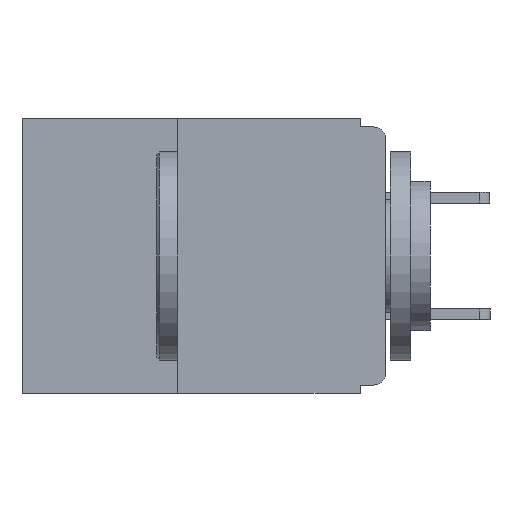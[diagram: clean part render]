
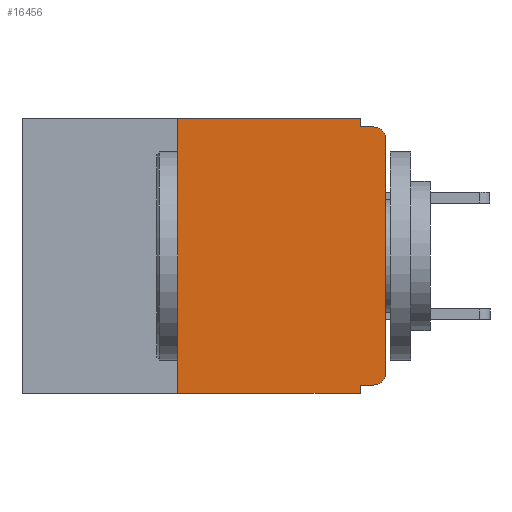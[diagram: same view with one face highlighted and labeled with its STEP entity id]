
A CAD part, left-side view. The second image highlights one B-rep face of the part: STEP entity #16456.
In plain terms, the highlighted planar face has unit normal (-1, 0, 0).
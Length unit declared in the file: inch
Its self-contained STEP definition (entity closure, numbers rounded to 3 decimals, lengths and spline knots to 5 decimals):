
#12 = EDGE_CURVE ( 'NONE', #5879, #13199, #8867, .T. ) ;
#127 = DIRECTION ( 'NONE',  ( -1., 0., 0. ) ) ;
#470 = CARTESIAN_POINT ( 'NONE',  ( 0., 0.031, -0.01 ) ) ;
#661 = CIRCLE ( 'NONE', #15094, 0.015 ) ;
#1228 = CARTESIAN_POINT ( 'NONE',  ( 0., 0.437, -0.33 ) ) ;
#1317 = DIRECTION ( 'NONE',  ( 1., 0., 0. ) ) ;
#1922 = VECTOR ( 'NONE', #11821, 39.37008 ) ;
#2860 = ORIENTED_EDGE ( 'NONE', *, *, #17256, .F. ) ;
#2930 = CARTESIAN_POINT ( 'NONE',  ( 0., 0., 0. ) ) ;
#3651 = VECTOR ( 'NONE', #21465, 39.37008 ) ;
#4110 = DIRECTION ( 'NONE',  ( 0., 0., -1. ) ) ;
#4394 = CARTESIAN_POINT ( 'NONE',  ( 0., 0.015, -0.025 ) ) ;
#4714 = CARTESIAN_POINT ( 'NONE',  ( 0., 0.015, -0.01 ) ) ;
#5103 = CARTESIAN_POINT ( 'NONE',  ( 0., 0.031, -0.33 ) ) ;
#5596 = CARTESIAN_POINT ( 'NONE',  ( 0., 0.25, -0.33 ) ) ;
#5879 = VERTEX_POINT ( 'NONE', #21097 ) ;
#6270 = VERTEX_POINT ( 'NONE', #7501 ) ;
#6344 = DIRECTION ( 'NONE',  ( 0., 0., -1. ) ) ;
#6626 = VECTOR ( 'NONE', #9047, 39.37008 ) ;
#7061 = CARTESIAN_POINT ( 'NONE',  ( 0., 0., -0.01 ) ) ;
#7126 = FACE_OUTER_BOUND ( 'NONE', #15646, .T. ) ;
#7146 = DIRECTION ( 'NONE',  ( 0., -1., 0. ) ) ;
#7501 = CARTESIAN_POINT ( 'NONE',  ( 0., 0., -0.305 ) ) ;
#7836 = EDGE_CURVE ( 'NONE', #10097, #23641, #9971, .T. ) ;
#7863 = CIRCLE ( 'NONE', #21084, 0.015 ) ;
#8867 = LINE ( 'NONE', #21626, #3651 ) ;
#8959 = LINE ( 'NONE', #16538, #19299 ) ;
#9010 = ORIENTED_EDGE ( 'NONE', *, *, #12, .F. ) ;
#9047 = DIRECTION ( 'NONE',  ( 0., -1., 0. ) ) ;
#9435 = EDGE_CURVE ( 'NONE', #13199, #20300, #24879, .T. ) ;
#9504 = DIRECTION ( 'NONE',  ( 0., 0., 1. ) ) ;
#9971 = LINE ( 'NONE', #7061, #24663 ) ;
#9978 = EDGE_CURVE ( 'NONE', #22343, #18645, #12930, .T. ) ;
#10097 = VERTEX_POINT ( 'NONE', #470 ) ;
#10645 = CARTESIAN_POINT ( 'NONE',  ( 0., 0., -0.025 ) ) ;
#10680 = DIRECTION ( 'NONE',  ( 0., 0., -1. ) ) ;
#11025 = PLANE ( 'NONE',  #11120 ) ;
#11120 = AXIS2_PLACEMENT_3D ( 'NONE', #24417, #1317, #14962 ) ;
#11288 = CARTESIAN_POINT ( 'NONE',  ( 0., 0.031, -0.32 ) ) ;
#11643 = VERTEX_POINT ( 'NONE', #20158 ) ;
#11813 = CARTESIAN_POINT ( 'NONE',  ( 0., 0.015, -0.305 ) ) ;
#11821 = DIRECTION ( 'NONE',  ( 0., -1., 0. ) ) ;
#11960 = ORIENTED_EDGE ( 'NONE', *, *, #9978, .F. ) ;
#12430 = LINE ( 'NONE', #2930, #13016 ) ;
#12455 = ORIENTED_EDGE ( 'NONE', *, *, #21321, .T. ) ;
#12930 = LINE ( 'NONE', #23226, #1922 ) ;
#13016 = VECTOR ( 'NONE', #16585, 39.37008 ) ;
#13199 = VERTEX_POINT ( 'NONE', #11288 ) ;
#13505 = ORIENTED_EDGE ( 'NONE', *, *, #15676, .T. ) ;
#13776 = DIRECTION ( 'NONE',  ( 0., 0., -1. ) ) ;
#14694 = EDGE_CURVE ( 'NONE', #11643, #20300, #22144, .T. ) ;
#14804 = VECTOR ( 'NONE', #4110, 39.37008 ) ;
#14962 = DIRECTION ( 'NONE',  ( 0., 0., -1. ) ) ;
#15094 = AXIS2_PLACEMENT_3D ( 'NONE', #11813, #127, #13776 ) ;
#15292 = CARTESIAN_POINT ( 'NONE',  ( 0., 0.031, 0. ) ) ;
#15646 = EDGE_LOOP ( 'NONE', ( #13505, #12455, #21933, #2860, #11960, #16201, #22421, #16078, #9010, #17825 ) ) ;
#15676 = EDGE_CURVE ( 'NONE', #6270, #23658, #12430, .T. ) ;
#15959 = EDGE_CURVE ( 'NONE', #11643, #22343, #21156, .T. ) ;
#16078 = ORIENTED_EDGE ( 'NONE', *, *, #9435, .F. ) ;
#16201 = ORIENTED_EDGE ( 'NONE', *, *, #15959, .F. ) ;
#16456 = ADVANCED_FACE ( 'NONE', ( #7126 ), #11025, .F. ) ;
#16538 = CARTESIAN_POINT ( 'NONE',  ( 0., 0.031, 0. ) ) ;
#16585 = DIRECTION ( 'NONE',  ( 0., 0., 1. ) ) ;
#16641 = VECTOR ( 'NONE', #9504, 39.37008 ) ;
#17256 = EDGE_CURVE ( 'NONE', #18645, #10097, #8959, .T. ) ;
#17825 = ORIENTED_EDGE ( 'NONE', *, *, #18745, .T. ) ;
#18056 = DIRECTION ( 'NONE',  ( -1., 0., 0. ) ) ;
#18645 = VERTEX_POINT ( 'NONE', #15292 ) ;
#18745 = EDGE_CURVE ( 'NONE', #5879, #6270, #661, .T. ) ;
#19299 = VECTOR ( 'NONE', #10680, 39.37008 ) ;
#20158 = CARTESIAN_POINT ( 'NONE',  ( 0., 0.25, -0.33 ) ) ;
#20300 = VERTEX_POINT ( 'NONE', #5103 ) ;
#21084 = AXIS2_PLACEMENT_3D ( 'NONE', #4394, #18056, #6344 ) ;
#21097 = CARTESIAN_POINT ( 'NONE',  ( 0., 0.015, -0.32 ) ) ;
#21156 = LINE ( 'NONE', #5596, #16641 ) ;
#21321 = EDGE_CURVE ( 'NONE', #23658, #23641, #7863, .T. ) ;
#21465 = DIRECTION ( 'NONE',  ( 0., 1., 0. ) ) ;
#21625 = CARTESIAN_POINT ( 'NONE',  ( 0., 0.031, -0.33 ) ) ;
#21626 = CARTESIAN_POINT ( 'NONE',  ( 0., 0., -0.32 ) ) ;
#21933 = ORIENTED_EDGE ( 'NONE', *, *, #7836, .F. ) ;
#22144 = LINE ( 'NONE', #1228, #6626 ) ;
#22343 = VERTEX_POINT ( 'NONE', #23246 ) ;
#22421 = ORIENTED_EDGE ( 'NONE', *, *, #14694, .T. ) ;
#23226 = CARTESIAN_POINT ( 'NONE',  ( 0., 0.437, 0. ) ) ;
#23246 = CARTESIAN_POINT ( 'NONE',  ( 0., 0.25, 0. ) ) ;
#23641 = VERTEX_POINT ( 'NONE', #4714 ) ;
#23658 = VERTEX_POINT ( 'NONE', #10645 ) ;
#24417 = CARTESIAN_POINT ( 'NONE',  ( 0., 0.437, 0. ) ) ;
#24663 = VECTOR ( 'NONE', #7146, 39.37008 ) ;
#24879 = LINE ( 'NONE', #21625, #14804 ) ;
